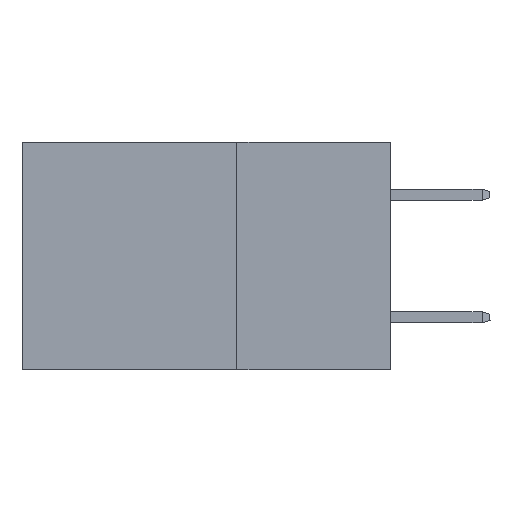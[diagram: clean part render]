
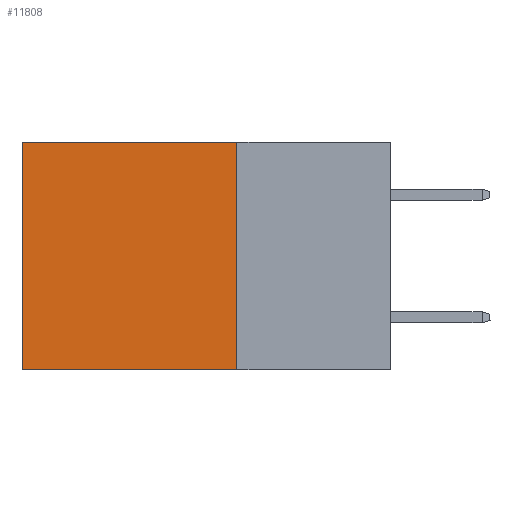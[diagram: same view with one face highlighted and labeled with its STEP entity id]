
A CAD part, left-side view. The second image highlights one B-rep face of the part: STEP entity #11808.
In plain terms, the highlighted planar face has unit normal (-1, 0, 0).
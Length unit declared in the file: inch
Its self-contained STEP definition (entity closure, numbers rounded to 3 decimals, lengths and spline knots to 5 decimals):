
#275 = DIRECTION ( 'NONE',  ( 0., 0., -1. ) ) ;
#293 = EDGE_CURVE ( 'NONE', #3655, #24166, #2003, .T. ) ;
#1460 = VECTOR ( 'NONE', #4242, 39.37008 ) ;
#2003 = LINE ( 'NONE', #5173, #18311 ) ;
#2559 = CARTESIAN_POINT ( 'NONE',  ( 0.2875, 0.25, 0. ) ) ;
#2630 = ORIENTED_EDGE ( 'NONE', *, *, #27196, .F. ) ;
#2647 = DIRECTION ( 'NONE',  ( 1., 0., 0. ) ) ;
#3330 = AXIS2_PLACEMENT_3D ( 'NONE', #2559, #2647, #18154 ) ;
#3655 = VERTEX_POINT ( 'NONE', #22747 ) ;
#4242 = DIRECTION ( 'NONE',  ( 0., 1., 0. ) ) ;
#5173 = CARTESIAN_POINT ( 'NONE',  ( 0.2875, 0.25, 0. ) ) ;
#6132 = CARTESIAN_POINT ( 'NONE',  ( 0.2875, 0.25, -0.37 ) ) ;
#6137 = CARTESIAN_POINT ( 'NONE',  ( 0.2875, 0.6, 0. ) ) ;
#6676 = ORIENTED_EDGE ( 'NONE', *, *, #293, .F. ) ;
#7418 = EDGE_CURVE ( 'NONE', #3655, #16798, #15215, .T. ) ;
#7622 = VECTOR ( 'NONE', #11407, 39.37008 ) ;
#8786 = CARTESIAN_POINT ( 'NONE',  ( 0.2875, 0.25, -0.37 ) ) ;
#9865 = VERTEX_POINT ( 'NONE', #10125 ) ;
#10125 = CARTESIAN_POINT ( 'NONE',  ( 0.2875, 0.6, -0.37 ) ) ;
#11407 = DIRECTION ( 'NONE',  ( 0., 0., -1. ) ) ;
#11587 = PLANE ( 'NONE',  #3330 ) ;
#11808 = ADVANCED_FACE ( 'NONE', ( #12965 ), #11587, .F. ) ;
#11975 = EDGE_LOOP ( 'NONE', ( #24806, #2630, #6676, #12584 ) ) ;
#12584 = ORIENTED_EDGE ( 'NONE', *, *, #7418, .T. ) ;
#12965 = FACE_OUTER_BOUND ( 'NONE', #11975, .T. ) ;
#13647 = DIRECTION ( 'NONE',  ( 0., 1., 0. ) ) ;
#15215 = LINE ( 'NONE', #26657, #19656 ) ;
#16798 = VERTEX_POINT ( 'NONE', #6137 ) ;
#17056 = EDGE_CURVE ( 'NONE', #16798, #9865, #19314, .T. ) ;
#18154 = DIRECTION ( 'NONE',  ( 0., 0., -1. ) ) ;
#18311 = VECTOR ( 'NONE', #275, 39.37008 ) ;
#19140 = LINE ( 'NONE', #8786, #1460 ) ;
#19314 = LINE ( 'NONE', #20060, #7622 ) ;
#19656 = VECTOR ( 'NONE', #13647, 39.37008 ) ;
#20060 = CARTESIAN_POINT ( 'NONE',  ( 0.2875, 0.6, 0. ) ) ;
#22747 = CARTESIAN_POINT ( 'NONE',  ( 0.2875, 0.25, 0. ) ) ;
#24166 = VERTEX_POINT ( 'NONE', #6132 ) ;
#24806 = ORIENTED_EDGE ( 'NONE', *, *, #17056, .T. ) ;
#26657 = CARTESIAN_POINT ( 'NONE',  ( 0.2875, 0.25, 0. ) ) ;
#27196 = EDGE_CURVE ( 'NONE', #24166, #9865, #19140, .T. ) ;
